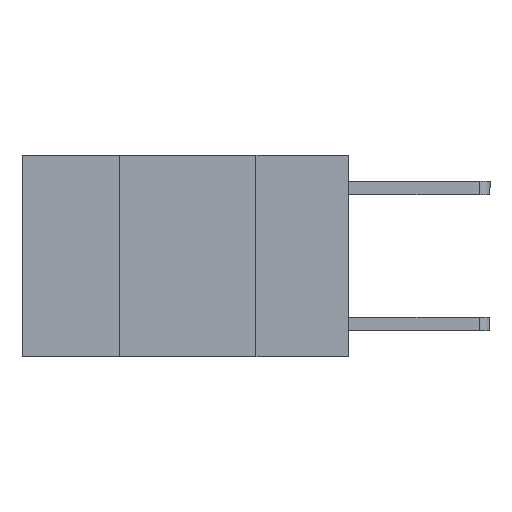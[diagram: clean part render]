
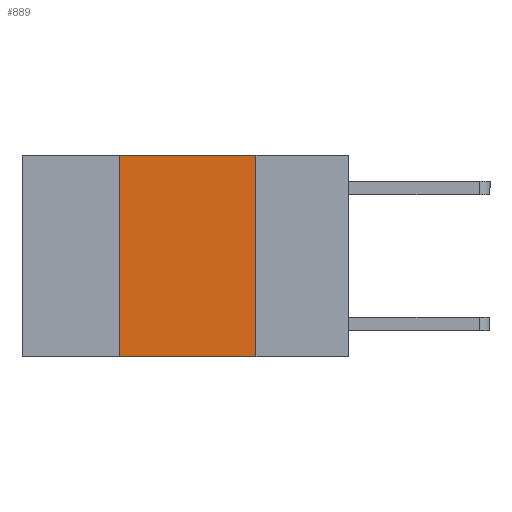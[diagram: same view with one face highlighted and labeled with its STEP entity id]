
A CAD part, left-side view. The second image highlights one B-rep face of the part: STEP entity #889.
In plain terms, the highlighted planar face has unit normal (-1, 0, 0).
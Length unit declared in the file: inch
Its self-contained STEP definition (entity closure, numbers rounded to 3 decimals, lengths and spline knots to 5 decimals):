
#216 = DIRECTION ( 'NONE',  ( 1., 0., 0. ) ) ;
#269 = DIRECTION ( 'NONE',  ( 0., 0., -1. ) ) ;
#352 = CARTESIAN_POINT ( 'NONE',  ( 0., 0.6, 0. ) ) ;
#404 = CARTESIAN_POINT ( 'NONE',  ( 0., 0.6, 0. ) ) ;
#491 = EDGE_CURVE ( 'NONE', #6389, #7601, #3551, .T. ) ;
#889 = ADVANCED_FACE ( 'NONE', ( #6485 ), #3716, .F. ) ;
#934 = EDGE_CURVE ( 'NONE', #6996, #5422, #7068, .T. ) ;
#1350 = VECTOR ( 'NONE', #7016, 39.37008 ) ;
#1503 = AXIS2_PLACEMENT_3D ( 'NONE', #352, #216, #269 ) ;
#1560 = DIRECTION ( 'NONE',  ( 0., -1., 0. ) ) ;
#2053 = EDGE_CURVE ( 'NONE', #5422, #7601, #5258, .T. ) ;
#2083 = CARTESIAN_POINT ( 'NONE',  ( 0., 0.42, 0. ) ) ;
#2314 = CARTESIAN_POINT ( 'NONE',  ( 0., 0.42, 0. ) ) ;
#2541 = EDGE_LOOP ( 'NONE', ( #6663, #6743, #4145, #6845 ) ) ;
#2873 = DIRECTION ( 'NONE',  ( 0., -1., 0. ) ) ;
#3216 = CARTESIAN_POINT ( 'NONE',  ( 0., 0.17, 0. ) ) ;
#3380 = VECTOR ( 'NONE', #2873, 39.37008 ) ;
#3551 = LINE ( 'NONE', #4991, #3380 ) ;
#3716 = PLANE ( 'NONE',  #1503 ) ;
#4145 = ORIENTED_EDGE ( 'NONE', *, *, #8011, .F. ) ;
#4863 = LINE ( 'NONE', #2083, #1350 ) ;
#4991 = CARTESIAN_POINT ( 'NONE',  ( 0., 0.6, -0.37 ) ) ;
#5258 = LINE ( 'NONE', #7983, #6256 ) ;
#5422 = VERTEX_POINT ( 'NONE', #3216 ) ;
#6256 = VECTOR ( 'NONE', #8765, 39.37008 ) ;
#6389 = VERTEX_POINT ( 'NONE', #7712 ) ;
#6485 = FACE_OUTER_BOUND ( 'NONE', #2541, .T. ) ;
#6663 = ORIENTED_EDGE ( 'NONE', *, *, #2053, .F. ) ;
#6743 = ORIENTED_EDGE ( 'NONE', *, *, #934, .F. ) ;
#6845 = ORIENTED_EDGE ( 'NONE', *, *, #491, .T. ) ;
#6996 = VERTEX_POINT ( 'NONE', #2314 ) ;
#7016 = DIRECTION ( 'NONE',  ( 0., 0., 1. ) ) ;
#7068 = LINE ( 'NONE', #404, #8497 ) ;
#7326 = CARTESIAN_POINT ( 'NONE',  ( 0., 0.17, -0.37 ) ) ;
#7601 = VERTEX_POINT ( 'NONE', #7326 ) ;
#7712 = CARTESIAN_POINT ( 'NONE',  ( 0., 0.42, -0.37 ) ) ;
#7983 = CARTESIAN_POINT ( 'NONE',  ( 0., 0.17, 0. ) ) ;
#8011 = EDGE_CURVE ( 'NONE', #6389, #6996, #4863, .T. ) ;
#8497 = VECTOR ( 'NONE', #1560, 39.37008 ) ;
#8765 = DIRECTION ( 'NONE',  ( 0., 0., -1. ) ) ;
